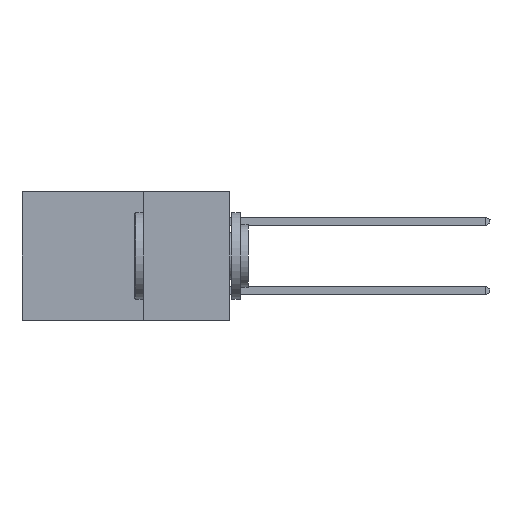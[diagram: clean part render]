
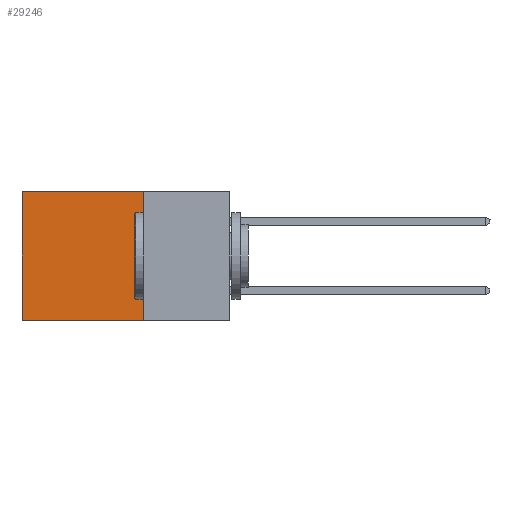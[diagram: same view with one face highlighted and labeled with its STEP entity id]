
A CAD part, left-side view. The second image highlights one B-rep face of the part: STEP entity #29246.
In plain terms, the highlighted planar face has unit normal (-1, 0, 0).
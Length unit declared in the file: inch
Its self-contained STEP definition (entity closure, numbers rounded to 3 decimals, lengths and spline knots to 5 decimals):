
#235 = VECTOR ( 'NONE', #17119, 39.37008 ) ;
#1337 = AXIS2_PLACEMENT_3D ( 'NONE', #1477, #29120, #26620 ) ;
#1477 = CARTESIAN_POINT ( 'NONE',  ( 0.298, 0.25, 0. ) ) ;
#2774 = DIRECTION ( 'NONE',  ( 0., 1., 0. ) ) ;
#6357 = LINE ( 'NONE', #19513, #12171 ) ;
#6434 = LINE ( 'NONE', #26189, #11067 ) ;
#6674 = PLANE ( 'NONE',  #1337 ) ;
#6814 = CARTESIAN_POINT ( 'NONE',  ( 0.298, 0.25, -0.37 ) ) ;
#6824 = LINE ( 'NONE', #29338, #235 ) ;
#7776 = VECTOR ( 'NONE', #2774, 39.37008 ) ;
#9173 = CARTESIAN_POINT ( 'NONE',  ( 0.298, 0.6, 0. ) ) ;
#11067 = VECTOR ( 'NONE', #18602, 39.37008 ) ;
#11680 = ORIENTED_EDGE ( 'NONE', *, *, #24406, .T. ) ;
#12171 = VECTOR ( 'NONE', #15419, 39.37008 ) ;
#12648 = CARTESIAN_POINT ( 'NONE',  ( 0.298, 0.25, -0.37 ) ) ;
#12908 = ORIENTED_EDGE ( 'NONE', *, *, #30335, .F. ) ;
#15419 = DIRECTION ( 'NONE',  ( 0., 0., -1. ) ) ;
#17119 = DIRECTION ( 'NONE',  ( 0., 0., -1. ) ) ;
#17294 = ORIENTED_EDGE ( 'NONE', *, *, #31102, .T. ) ;
#18602 = DIRECTION ( 'NONE',  ( 0., 1., 0. ) ) ;
#19513 = CARTESIAN_POINT ( 'NONE',  ( 0.298, 0.6, 0. ) ) ;
#20279 = EDGE_LOOP ( 'NONE', ( #11680, #12908, #31686, #17294 ) ) ;
#20437 = VERTEX_POINT ( 'NONE', #29292 ) ;
#21880 = CARTESIAN_POINT ( 'NONE',  ( 0.298, 0.6, -0.37 ) ) ;
#24406 = EDGE_CURVE ( 'NONE', #29313, #26555, #6357, .T. ) ;
#24872 = EDGE_CURVE ( 'NONE', #20437, #26567, #6824, .T. ) ;
#26189 = CARTESIAN_POINT ( 'NONE',  ( 0.298, 0.25, 0. ) ) ;
#26555 = VERTEX_POINT ( 'NONE', #21880 ) ;
#26567 = VERTEX_POINT ( 'NONE', #6814 ) ;
#26620 = DIRECTION ( 'NONE',  ( 0., 0., -1. ) ) ;
#26709 = LINE ( 'NONE', #12648, #7776 ) ;
#28753 = FACE_OUTER_BOUND ( 'NONE', #20279, .T. ) ;
#29120 = DIRECTION ( 'NONE',  ( 1., 0., 0. ) ) ;
#29246 = ADVANCED_FACE ( 'NONE', ( #28753 ), #6674, .F. ) ;
#29292 = CARTESIAN_POINT ( 'NONE',  ( 0.298, 0.25, 0. ) ) ;
#29313 = VERTEX_POINT ( 'NONE', #9173 ) ;
#29338 = CARTESIAN_POINT ( 'NONE',  ( 0.298, 0.25, 0. ) ) ;
#30335 = EDGE_CURVE ( 'NONE', #26567, #26555, #26709, .T. ) ;
#31102 = EDGE_CURVE ( 'NONE', #20437, #29313, #6434, .T. ) ;
#31686 = ORIENTED_EDGE ( 'NONE', *, *, #24872, .F. ) ;
